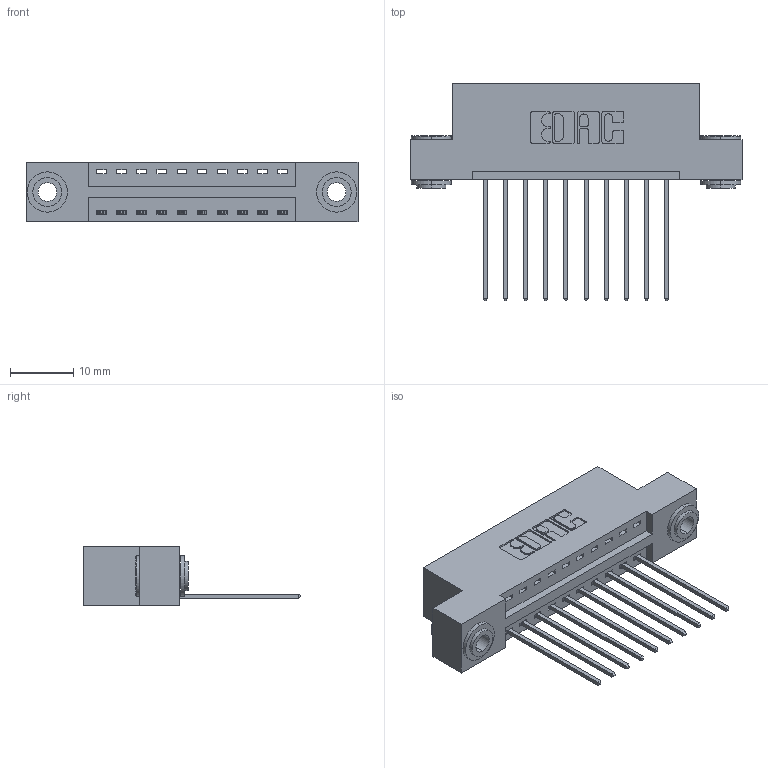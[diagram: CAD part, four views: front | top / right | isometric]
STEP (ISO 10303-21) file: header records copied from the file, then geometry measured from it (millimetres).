
FILE_DESCRIPTION (( 'STEP AP203' ), '1' );
FILE_NAME ('396-010-541-103.STEP', '2019-10-26T14:33:18', ( '' ), ( '' ), 'SwSTEP 2.0', 'SolidWorks 2016', '' );
FILE_SCHEMA (( 'CONFIG_CONTROL_DESIGN' ));
Length unit declared in the file: inch
Products named in the file (4): 396-010-541-103; 345-250-002_345-250-002-102; 345-292-001_345-293-141; 346 Part_Flush Mounting Lugs - 0.156 Dia-TH
Assembly tree (13 placements, depth 2):
  396-010-541-103
    346 Part_Flush Mounting Lugs - 0.156 Dia-TH
    345-292-001_345-293-141  x10
    345-250-002_345-250-002-102  x2
Bounding box: 52.32 x 34.29 x 9.4 mm (x, y, z)
Volume: 4840.5 mm3; surface area: 6121 mm2
Topology: 13 solids, 13 shells, 740 faces, 2165 edges, 1426 vertices
Faces by surface type: plane 486, cylinder 246, cone 8
Entity records: 11182 total; most frequent: CARTESIAN_POINT 1905, ORIENTED_EDGE 1842, DIRECTION 1751, EDGE_CURVE 921, LINE 725, VECTOR 725, VERTEX_POINT 610, AXIS2_PLACEMENT_3D 513
